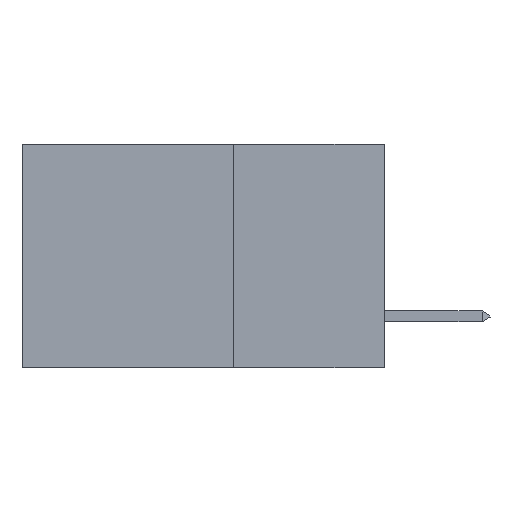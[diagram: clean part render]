
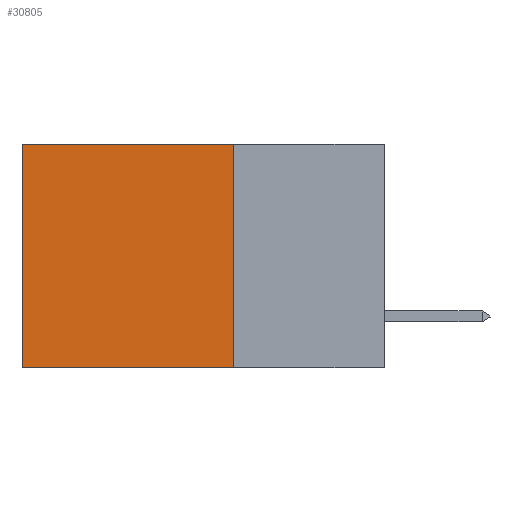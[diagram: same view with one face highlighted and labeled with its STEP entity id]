
A CAD part, left-side view. The second image highlights one B-rep face of the part: STEP entity #30805.
In plain terms, the highlighted planar face has unit normal (-1, 0, 0).
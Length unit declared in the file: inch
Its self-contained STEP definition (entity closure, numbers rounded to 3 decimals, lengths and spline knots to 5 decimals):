
#716 = EDGE_CURVE ( 'NONE', #13554, #48923, #17078, .T. ) ;
#1193 = DIRECTION ( 'NONE',  ( 0., 0., -1. ) ) ;
#1441 = AXIS2_PLACEMENT_3D ( 'NONE', #30741, #49935, #15190 ) ;
#1669 = ORIENTED_EDGE ( 'NONE', *, *, #716, .T. ) ;
#1976 = DIRECTION ( 'NONE',  ( 0., 1., 0. ) ) ;
#3032 = DIRECTION ( 'NONE',  ( 0., 1., 0. ) ) ;
#3935 = CARTESIAN_POINT ( 'NONE',  ( 0.2875, 0.25, -0.37 ) ) ;
#4937 = EDGE_CURVE ( 'NONE', #6076, #15498, #33989, .T. ) ;
#5186 = FACE_OUTER_BOUND ( 'NONE', #13587, .T. ) ;
#5832 = ORIENTED_EDGE ( 'NONE', *, *, #47899, .F. ) ;
#6076 = VERTEX_POINT ( 'NONE', #3935 ) ;
#6794 = CARTESIAN_POINT ( 'NONE',  ( 0.2875, 0.25, 0. ) ) ;
#9053 = LINE ( 'NONE', #43872, #41342 ) ;
#13554 = VERTEX_POINT ( 'NONE', #36687 ) ;
#13587 = EDGE_LOOP ( 'NONE', ( #33820, #22340, #5832, #1669 ) ) ;
#15190 = DIRECTION ( 'NONE',  ( 0., 0., -1. ) ) ;
#15345 = VECTOR ( 'NONE', #3032, 39.37008 ) ;
#15498 = VERTEX_POINT ( 'NONE', #28654 ) ;
#16237 = EDGE_CURVE ( 'NONE', #48923, #15498, #36109, .T. ) ;
#17078 = LINE ( 'NONE', #6794, #15345 ) ;
#18259 = VECTOR ( 'NONE', #1976, 39.37008 ) ;
#22340 = ORIENTED_EDGE ( 'NONE', *, *, #4937, .F. ) ;
#22434 = PLANE ( 'NONE',  #1441 ) ;
#28654 = CARTESIAN_POINT ( 'NONE',  ( 0.2875, 0.6, -0.37 ) ) ;
#30693 = CARTESIAN_POINT ( 'NONE',  ( 0.2875, 0.25, -0.37 ) ) ;
#30741 = CARTESIAN_POINT ( 'NONE',  ( 0.2875, 0.25, 0. ) ) ;
#30805 = ADVANCED_FACE ( 'NONE', ( #5186 ), #22434, .F. ) ;
#33820 = ORIENTED_EDGE ( 'NONE', *, *, #16237, .T. ) ;
#33989 = LINE ( 'NONE', #30693, #18259 ) ;
#34384 = VECTOR ( 'NONE', #40030, 39.37008 ) ;
#35760 = CARTESIAN_POINT ( 'NONE',  ( 0.2875, 0.6, 0. ) ) ;
#36109 = LINE ( 'NONE', #35760, #34384 ) ;
#36687 = CARTESIAN_POINT ( 'NONE',  ( 0.2875, 0.25, 0. ) ) ;
#40030 = DIRECTION ( 'NONE',  ( 0., 0., -1. ) ) ;
#41342 = VECTOR ( 'NONE', #1193, 39.37008 ) ;
#41684 = CARTESIAN_POINT ( 'NONE',  ( 0.2875, 0.6, 0. ) ) ;
#43872 = CARTESIAN_POINT ( 'NONE',  ( 0.2875, 0.25, 0. ) ) ;
#47899 = EDGE_CURVE ( 'NONE', #13554, #6076, #9053, .T. ) ;
#48923 = VERTEX_POINT ( 'NONE', #41684 ) ;
#49935 = DIRECTION ( 'NONE',  ( 1., 0., 0. ) ) ;
